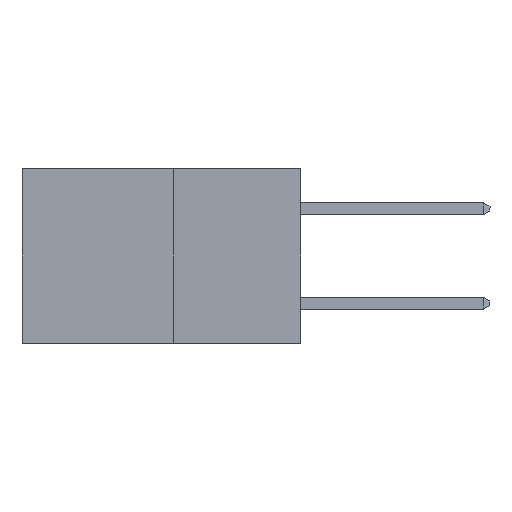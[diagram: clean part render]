
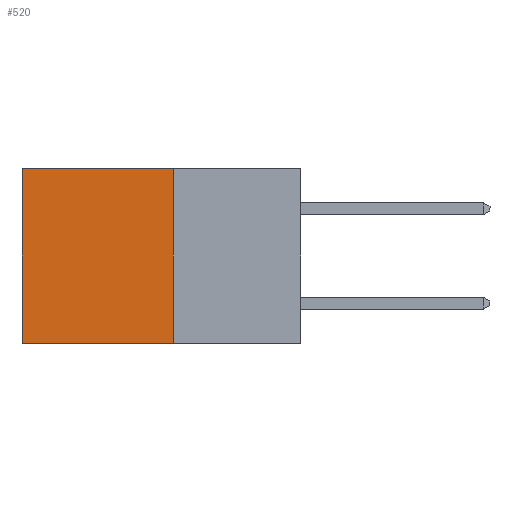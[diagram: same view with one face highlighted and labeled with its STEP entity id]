
A CAD part, left-side view. The second image highlights one B-rep face of the part: STEP entity #520.
In plain terms, the highlighted planar face has unit normal (-1, 0, 0).
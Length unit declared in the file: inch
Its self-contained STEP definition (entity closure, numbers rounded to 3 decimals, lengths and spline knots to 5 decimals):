
#520 = ADVANCED_FACE ( 'NONE', ( #2116 ), #7302, .F. ) ;
#826 = CARTESIAN_POINT ( 'NONE',  ( 0.277, 0.59, -0.37 ) ) ;
#1125 = EDGE_CURVE ( 'NONE', #6684, #4587, #7300, .T. ) ;
#1188 = VECTOR ( 'NONE', #3560, 39.37008 ) ;
#1299 = DIRECTION ( 'NONE',  ( 1., 0., 0. ) ) ;
#1706 = ORIENTED_EDGE ( 'NONE', *, *, #4409, .T. ) ;
#2116 = FACE_OUTER_BOUND ( 'NONE', #6594, .T. ) ;
#2406 = ORIENTED_EDGE ( 'NONE', *, *, #7604, .T. ) ;
#2675 = CARTESIAN_POINT ( 'NONE',  ( 0.277, 0.59, -0.37 ) ) ;
#2832 = CARTESIAN_POINT ( 'NONE',  ( 0.277, 0.27, -0.37 ) ) ;
#2940 = LINE ( 'NONE', #3629, #1188 ) ;
#2967 = CARTESIAN_POINT ( 'NONE',  ( 0.277, 0.27, -0.37 ) ) ;
#3553 = VECTOR ( 'NONE', #4020, 39.37008 ) ;
#3560 = DIRECTION ( 'NONE',  ( 0., 1., 0. ) ) ;
#3629 = CARTESIAN_POINT ( 'NONE',  ( 0.277, 0.27, 0. ) ) ;
#3656 = EDGE_CURVE ( 'NONE', #5796, #6684, #4890, .T. ) ;
#4020 = DIRECTION ( 'NONE',  ( 0., 1., 0. ) ) ;
#4274 = CARTESIAN_POINT ( 'NONE',  ( 0.277, 0.27, 0. ) ) ;
#4409 = EDGE_CURVE ( 'NONE', #8417, #4587, #6560, .T. ) ;
#4587 = VERTEX_POINT ( 'NONE', #2675 ) ;
#4774 = VECTOR ( 'NONE', #7500, 39.37008 ) ;
#4890 = LINE ( 'NONE', #2832, #7950 ) ;
#5089 = DIRECTION ( 'NONE',  ( 0., 0., -1. ) ) ;
#5195 = DIRECTION ( 'NONE',  ( 0., 0., -1. ) ) ;
#5796 = VERTEX_POINT ( 'NONE', #4274 ) ;
#6228 = CARTESIAN_POINT ( 'NONE',  ( 0.277, 0.27, -0.37 ) ) ;
#6560 = LINE ( 'NONE', #826, #4774 ) ;
#6594 = EDGE_LOOP ( 'NONE', ( #1706, #7997, #6903, #2406 ) ) ;
#6684 = VERTEX_POINT ( 'NONE', #2967 ) ;
#6818 = AXIS2_PLACEMENT_3D ( 'NONE', #7030, #1299, #5089 ) ;
#6903 = ORIENTED_EDGE ( 'NONE', *, *, #3656, .F. ) ;
#7030 = CARTESIAN_POINT ( 'NONE',  ( 0.277, 0.27, -0.37 ) ) ;
#7300 = LINE ( 'NONE', #6228, #3553 ) ;
#7302 = PLANE ( 'NONE',  #6818 ) ;
#7500 = DIRECTION ( 'NONE',  ( 0., 0., -1. ) ) ;
#7604 = EDGE_CURVE ( 'NONE', #5796, #8417, #2940, .T. ) ;
#7950 = VECTOR ( 'NONE', #5195, 39.37008 ) ;
#7997 = ORIENTED_EDGE ( 'NONE', *, *, #1125, .F. ) ;
#8417 = VERTEX_POINT ( 'NONE', #8450 ) ;
#8450 = CARTESIAN_POINT ( 'NONE',  ( 0.277, 0.59, 0. ) ) ;
